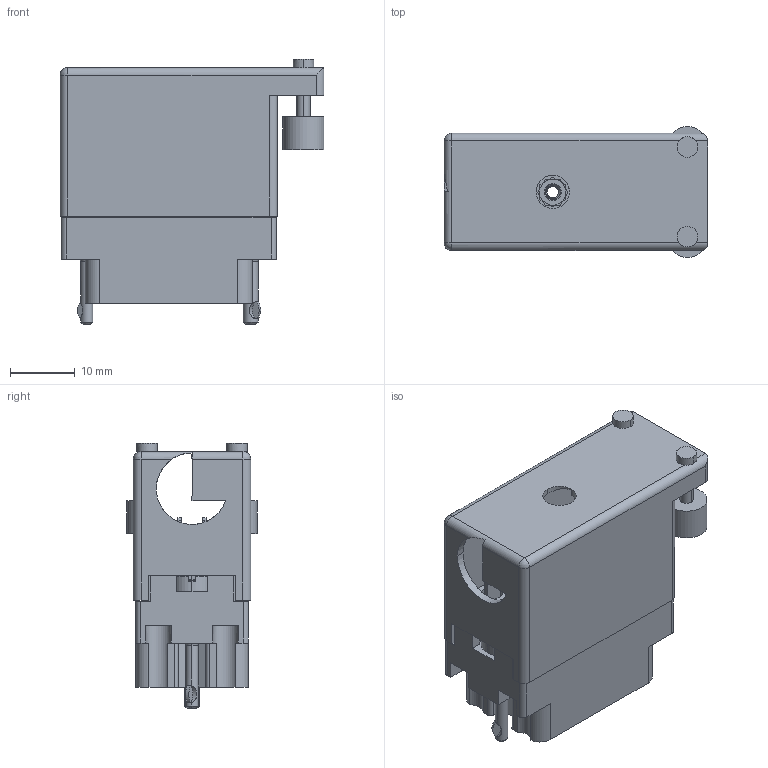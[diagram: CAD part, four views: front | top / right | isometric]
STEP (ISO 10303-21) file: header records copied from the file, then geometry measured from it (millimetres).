
FILE_DESCRIPTION (( 'STEP AP203' ), '1' );
FILE_NAME ('516-020-501-122.STEP', '2020-09-07T00:44:35', ( '' ), ( '' ), 'SwSTEP 2.0', 'SolidWorks 2020', '' );
FILE_SCHEMA (( 'CONFIG_CONTROL_DESIGN' ));
Length unit declared in the file: inch
Products named in the file (8): 516-230-001_Plastic - 020 Side Entry; 516-020-501-122; 516-292-001_501 Contact; 516-222-020-102_020; 516-252-021-102_020; 516 Plug Insulator_020; 516-222-020-102_021; 516-252-025-100_516-252-025-100
Assembly tree (27 placements, depth 2):
  516-020-501-122
    516 Plug Insulator_020
    516-292-001_501 Contact  x20
    516-230-001_Plastic - 020 Side Entry
    516-252-021-102_020  x2
    516-222-020-102_020
    516-252-025-100_516-252-025-100
    516-222-020-102_021
Bounding box: 40.87 x 20.24 x 41.1 mm (x, y, z)
Volume: 9364.2 mm3; surface area: 17759.2 mm2
Topology: 27 solids, 27 shells, 2366 faces, 6795 edges, 4491 vertices
Faces by surface type: plane 1341, cylinder 811, bspline 159, cone 49, torus 4, sphere 2
Entity records: 40016 total; most frequent: CARTESIAN_POINT 13362, ORIENTED_EDGE 5502, DIRECTION 5100, EDGE_CURVE 2751, VERTEX_POINT 1809, VECTOR 1766, LINE 1766, AXIS2_PLACEMENT_3D 1667
